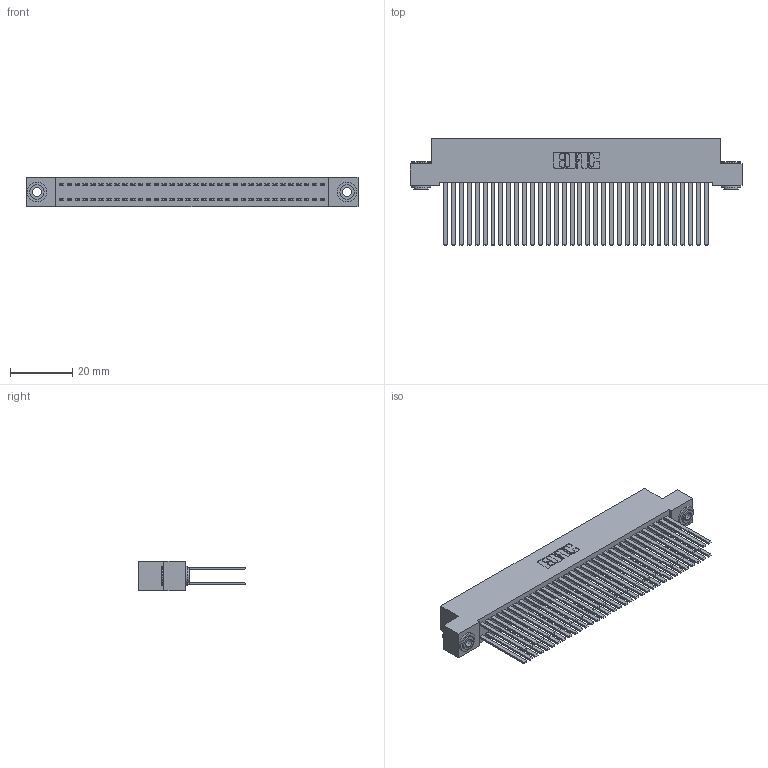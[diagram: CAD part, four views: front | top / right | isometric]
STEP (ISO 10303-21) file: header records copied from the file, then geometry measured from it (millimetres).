
FILE_DESCRIPTION (( 'STEP AP203' ), '1' );
FILE_NAME ('392-068-544-203.STEP', '2018-08-17T22:56:45', ( '' ), ( '' ), 'SwSTEP 2.0', 'SolidWorks 2016', '' );
FILE_SCHEMA (( 'CONFIG_CONTROL_DESIGN' ));
Length unit declared in the file: inch
Products named in the file (4): 342 Part_.156 TH; 345-292-001_345-293-144; 342-250-002_345-250-002-102; 392-068-544-203
Assembly tree (71 placements, depth 2):
  392-068-544-203
    342 Part_.156 TH
    345-292-001_345-293-144  x68
    342-250-002_345-250-002-102  x2
Bounding box: 106.68 x 34.3 x 9.4 mm (x, y, z)
Volume: 10523.4 mm3; surface area: 19786.2 mm2
Topology: 71 solids, 71 shells, 3276 faces, 9691 edges, 6366 vertices
Faces by surface type: plane 2252, cylinder 1016, cone 8
Entity records: 23242 total; most frequent: CARTESIAN_POINT 3833, ORIENTED_EDGE 3762, DIRECTION 3319, EDGE_CURVE 1881, VECTOR 1733, LINE 1733, VERTEX_POINT 1250, AXIS2_PLACEMENT_3D 793
